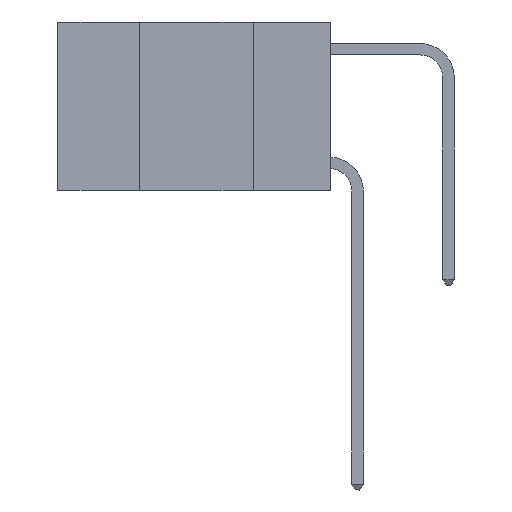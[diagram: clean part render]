
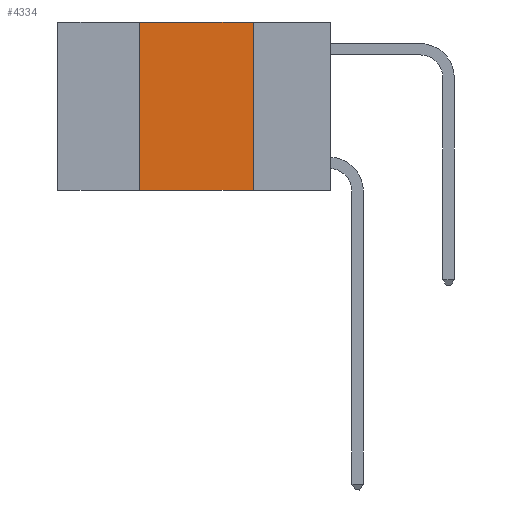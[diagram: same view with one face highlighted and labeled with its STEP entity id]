
A CAD part, left-side view. The second image highlights one B-rep face of the part: STEP entity #4334.
In plain terms, the highlighted planar face has unit normal (-1, 0, 0).
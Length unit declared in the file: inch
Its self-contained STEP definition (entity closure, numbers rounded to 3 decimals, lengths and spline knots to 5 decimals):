
#57 = CARTESIAN_POINT ( 'NONE',  ( 0., 0.42, -0.37 ) ) ;
#201 = VERTEX_POINT ( 'NONE', #5324 ) ;
#681 = VECTOR ( 'NONE', #720, 39.37008 ) ;
#697 = ORIENTED_EDGE ( 'NONE', *, *, #9018, .T. ) ;
#720 = DIRECTION ( 'NONE',  ( 0., 0., -1. ) ) ;
#1642 = VECTOR ( 'NONE', #11545, 39.37008 ) ;
#2322 = CARTESIAN_POINT ( 'NONE',  ( 0., 0.17, 0. ) ) ;
#2484 = VERTEX_POINT ( 'NONE', #2322 ) ;
#2648 = ORIENTED_EDGE ( 'NONE', *, *, #12149, .F. ) ;
#3206 = VERTEX_POINT ( 'NONE', #57 ) ;
#3378 = CARTESIAN_POINT ( 'NONE',  ( 0., 0.6, -0.37 ) ) ;
#3487 = CARTESIAN_POINT ( 'NONE',  ( 0., 0.6, 0. ) ) ;
#3511 = DIRECTION ( 'NONE',  ( 0., 0., 1. ) ) ;
#3533 = DIRECTION ( 'NONE',  ( 0., 0., -1. ) ) ;
#4334 = ADVANCED_FACE ( 'NONE', ( #7814 ), #8693, .F. ) ;
#5324 = CARTESIAN_POINT ( 'NONE',  ( 0., 0.42, 0. ) ) ;
#6342 = EDGE_CURVE ( 'NONE', #2484, #7279, #6526, .T. ) ;
#6526 = LINE ( 'NONE', #11202, #681 ) ;
#6909 = VECTOR ( 'NONE', #9933, 39.37008 ) ;
#7279 = VERTEX_POINT ( 'NONE', #8364 ) ;
#7290 = ORIENTED_EDGE ( 'NONE', *, *, #6342, .F. ) ;
#7814 = FACE_OUTER_BOUND ( 'NONE', #10250, .T. ) ;
#7920 = CARTESIAN_POINT ( 'NONE',  ( 0., 0.6, 0. ) ) ;
#8364 = CARTESIAN_POINT ( 'NONE',  ( 0., 0.17, -0.37 ) ) ;
#8448 = LINE ( 'NONE', #9684, #10785 ) ;
#8693 = PLANE ( 'NONE',  #11281 ) ;
#9018 = EDGE_CURVE ( 'NONE', #3206, #7279, #12696, .T. ) ;
#9339 = EDGE_CURVE ( 'NONE', #201, #2484, #12226, .T. ) ;
#9684 = CARTESIAN_POINT ( 'NONE',  ( 0., 0.42, 0. ) ) ;
#9706 = DIRECTION ( 'NONE',  ( 1., 0., 0. ) ) ;
#9933 = DIRECTION ( 'NONE',  ( 0., -1., 0. ) ) ;
#10250 = EDGE_LOOP ( 'NONE', ( #7290, #13235, #2648, #697 ) ) ;
#10785 = VECTOR ( 'NONE', #3511, 39.37008 ) ;
#11202 = CARTESIAN_POINT ( 'NONE',  ( 0., 0.17, 0. ) ) ;
#11281 = AXIS2_PLACEMENT_3D ( 'NONE', #3487, #9706, #3533 ) ;
#11545 = DIRECTION ( 'NONE',  ( 0., -1., 0. ) ) ;
#12149 = EDGE_CURVE ( 'NONE', #3206, #201, #8448, .T. ) ;
#12226 = LINE ( 'NONE', #7920, #6909 ) ;
#12696 = LINE ( 'NONE', #3378, #1642 ) ;
#13235 = ORIENTED_EDGE ( 'NONE', *, *, #9339, .F. ) ;
